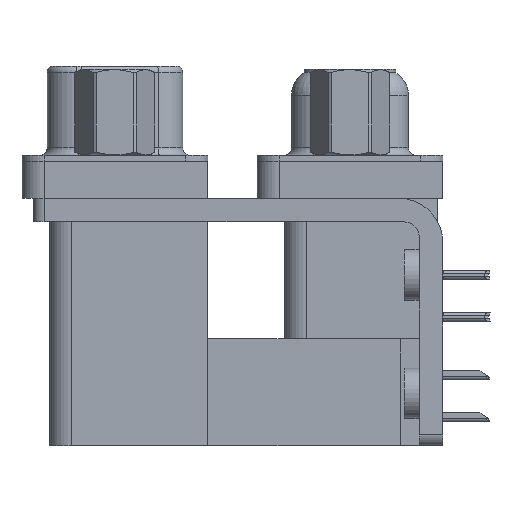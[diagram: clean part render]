
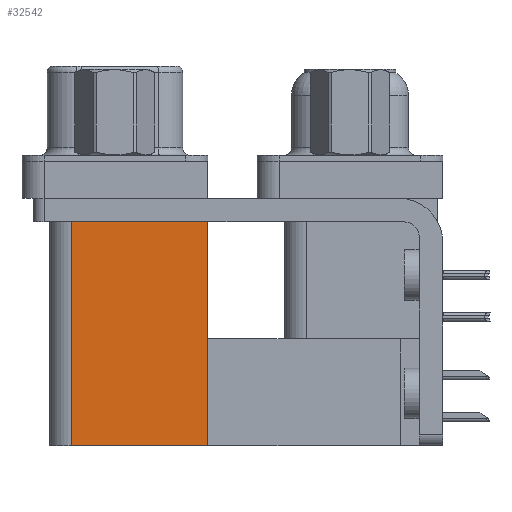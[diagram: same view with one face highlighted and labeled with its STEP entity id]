
A CAD part, left-side view. The second image highlights one B-rep face of the part: STEP entity #32542.
In plain terms, the highlighted planar face has unit normal (-1, 0, 0).
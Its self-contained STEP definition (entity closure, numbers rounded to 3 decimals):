
#872 = ORIENTED_EDGE ( 'NONE', *, *, #10793, .T. ) ;
#1352 = VERTEX_POINT ( 'NONE', #5341 ) ;
#1439 = CARTESIAN_POINT ( 'NONE',  ( 3.765, 9.6, -2.5 ) ) ;
#2305 = ORIENTED_EDGE ( 'NONE', *, *, #28406, .F. ) ;
#5341 = CARTESIAN_POINT ( 'NONE',  ( 3.765, 18.8, -2.5 ) ) ;
#6093 = LINE ( 'NONE', #37705, #30797 ) ;
#6337 = DIRECTION ( 'NONE',  ( 0., 0., 1. ) ) ;
#9047 = CARTESIAN_POINT ( 'NONE',  ( 3.765, 9.6, -19.2 ) ) ;
#10018 = AXIS2_PLACEMENT_3D ( 'NONE', #9047, #24800, #40653 ) ;
#10793 = EDGE_CURVE ( 'NONE', #43573, #1352, #33492, .T. ) ;
#11051 = CARTESIAN_POINT ( 'NONE',  ( 3.765, 9.6, -19.2 ) ) ;
#12899 = PLANE ( 'NONE',  #10018 ) ;
#13164 = LINE ( 'NONE', #48972, #33451 ) ;
#13736 = VECTOR ( 'NONE', #24915, 1000. ) ;
#14403 = LINE ( 'NONE', #11051, #31256 ) ;
#17585 = CARTESIAN_POINT ( 'NONE',  ( 3.765, 9.6, -19.2 ) ) ;
#20548 = EDGE_LOOP ( 'NONE', ( #872, #47698, #2305, #33326 ) ) ;
#24800 = DIRECTION ( 'NONE',  ( 1., 0., 0. ) ) ;
#24915 = DIRECTION ( 'NONE',  ( 0., 1., 0. ) ) ;
#25399 = CARTESIAN_POINT ( 'NONE',  ( 3.765, 9.6, -2.5 ) ) ;
#28406 = EDGE_CURVE ( 'NONE', #47967, #46791, #14403, .T. ) ;
#28464 = DIRECTION ( 'NONE',  ( 0., 0., 1. ) ) ;
#30797 = VECTOR ( 'NONE', #6337, 1000. ) ;
#31256 = VECTOR ( 'NONE', #41652, 1000. ) ;
#32542 = ADVANCED_FACE ( 'NONE', ( #36524 ), #12899, .F. ) ;
#33326 = ORIENTED_EDGE ( 'NONE', *, *, #36214, .T. ) ;
#33451 = VECTOR ( 'NONE', #28464, 1000. ) ;
#33492 = LINE ( 'NONE', #25399, #13736 ) ;
#34691 = CARTESIAN_POINT ( 'NONE',  ( 3.765, 18.8, -19.2 ) ) ;
#36214 = EDGE_CURVE ( 'NONE', #47967, #43573, #6093, .T. ) ;
#36524 = FACE_OUTER_BOUND ( 'NONE', #20548, .T. ) ;
#37705 = CARTESIAN_POINT ( 'NONE',  ( 3.765, 9.6, -19.2 ) ) ;
#40653 = DIRECTION ( 'NONE',  ( 0., 0., -1. ) ) ;
#41566 = EDGE_CURVE ( 'NONE', #46791, #1352, #13164, .T. ) ;
#41652 = DIRECTION ( 'NONE',  ( 0., 1., 0. ) ) ;
#43573 = VERTEX_POINT ( 'NONE', #1439 ) ;
#46791 = VERTEX_POINT ( 'NONE', #34691 ) ;
#47698 = ORIENTED_EDGE ( 'NONE', *, *, #41566, .F. ) ;
#47967 = VERTEX_POINT ( 'NONE', #17585 ) ;
#48972 = CARTESIAN_POINT ( 'NONE',  ( 3.765, 18.8, -19.2 ) ) ;
